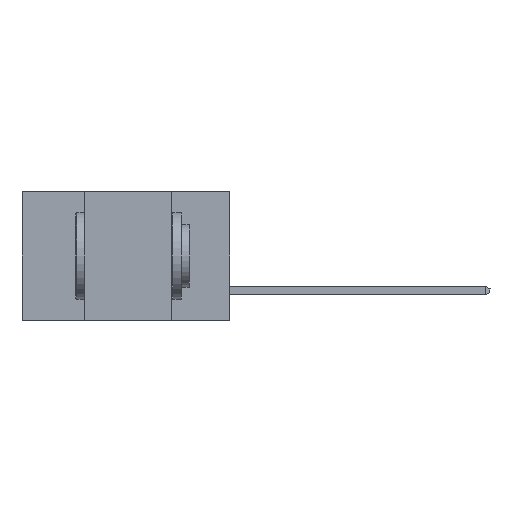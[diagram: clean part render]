
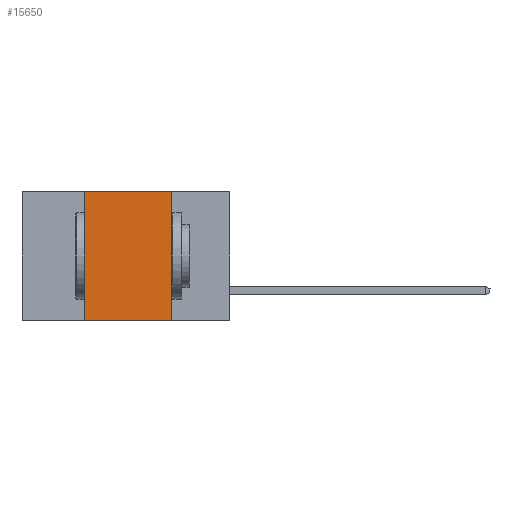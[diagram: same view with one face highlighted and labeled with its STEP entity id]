
A CAD part, left-side view. The second image highlights one B-rep face of the part: STEP entity #15650.
In plain terms, the highlighted planar face has unit normal (-1, 0, 0).
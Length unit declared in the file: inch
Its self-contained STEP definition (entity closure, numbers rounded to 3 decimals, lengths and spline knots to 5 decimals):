
#663 = CARTESIAN_POINT ( 'NONE',  ( 0., 0.42, -0.37 ) ) ;
#838 = LINE ( 'NONE', #9567, #12688 ) ;
#852 = LINE ( 'NONE', #16818, #8944 ) ;
#1259 = EDGE_CURVE ( 'NONE', #1796, #14092, #838, .T. ) ;
#1448 = CARTESIAN_POINT ( 'NONE',  ( 0., 0.6, 0. ) ) ;
#1796 = VERTEX_POINT ( 'NONE', #663 ) ;
#1926 = CARTESIAN_POINT ( 'NONE',  ( 0., 0.17, -0.37 ) ) ;
#3099 = CARTESIAN_POINT ( 'NONE',  ( 0., 0.17, -0.37 ) ) ;
#3758 = AXIS2_PLACEMENT_3D ( 'NONE', #1448, #5923, #17504 ) ;
#3870 = DIRECTION ( 'NONE',  ( 0., -1., 0. ) ) ;
#3886 = DIRECTION ( 'NONE',  ( 0., -1., 0. ) ) ;
#5161 = VECTOR ( 'NONE', #3886, 39.37008 ) ;
#5167 = ORIENTED_EDGE ( 'NONE', *, *, #1259, .F. ) ;
#5923 = DIRECTION ( 'NONE',  ( 1., 0., 0. ) ) ;
#6307 = ORIENTED_EDGE ( 'NONE', *, *, #9748, .F. ) ;
#6542 = EDGE_LOOP ( 'NONE', ( #6602, #6307, #5167, #16638 ) ) ;
#6602 = ORIENTED_EDGE ( 'NONE', *, *, #18565, .F. ) ;
#7153 = FACE_OUTER_BOUND ( 'NONE', #6542, .T. ) ;
#8370 = LINE ( 'NONE', #13782, #5161 ) ;
#8920 = DIRECTION ( 'NONE',  ( 0., 0., -1. ) ) ;
#8944 = VECTOR ( 'NONE', #3870, 39.37008 ) ;
#9567 = CARTESIAN_POINT ( 'NONE',  ( 0., 0.42, -0.37 ) ) ;
#9748 = EDGE_CURVE ( 'NONE', #14092, #10844, #8370, .T. ) ;
#10406 = VECTOR ( 'NONE', #8920, 39.37008 ) ;
#10844 = VERTEX_POINT ( 'NONE', #17606 ) ;
#10960 = VERTEX_POINT ( 'NONE', #1926 ) ;
#11533 = CARTESIAN_POINT ( 'NONE',  ( 0., 0.42, 0. ) ) ;
#11707 = PLANE ( 'NONE',  #3758 ) ;
#12688 = VECTOR ( 'NONE', #15364, 39.37008 ) ;
#13782 = CARTESIAN_POINT ( 'NONE',  ( 0., 0.6, 0. ) ) ;
#14092 = VERTEX_POINT ( 'NONE', #11533 ) ;
#15364 = DIRECTION ( 'NONE',  ( 0., 0., 1. ) ) ;
#15650 = ADVANCED_FACE ( 'NONE', ( #7153 ), #11707, .F. ) ;
#15752 = EDGE_CURVE ( 'NONE', #1796, #10960, #852, .T. ) ;
#16638 = ORIENTED_EDGE ( 'NONE', *, *, #15752, .T. ) ;
#16818 = CARTESIAN_POINT ( 'NONE',  ( 0., 0.6, -0.37 ) ) ;
#17504 = DIRECTION ( 'NONE',  ( 0., 0., -1. ) ) ;
#17606 = CARTESIAN_POINT ( 'NONE',  ( 0., 0.17, 0. ) ) ;
#17748 = LINE ( 'NONE', #3099, #10406 ) ;
#18565 = EDGE_CURVE ( 'NONE', #10844, #10960, #17748, .T. ) ;
